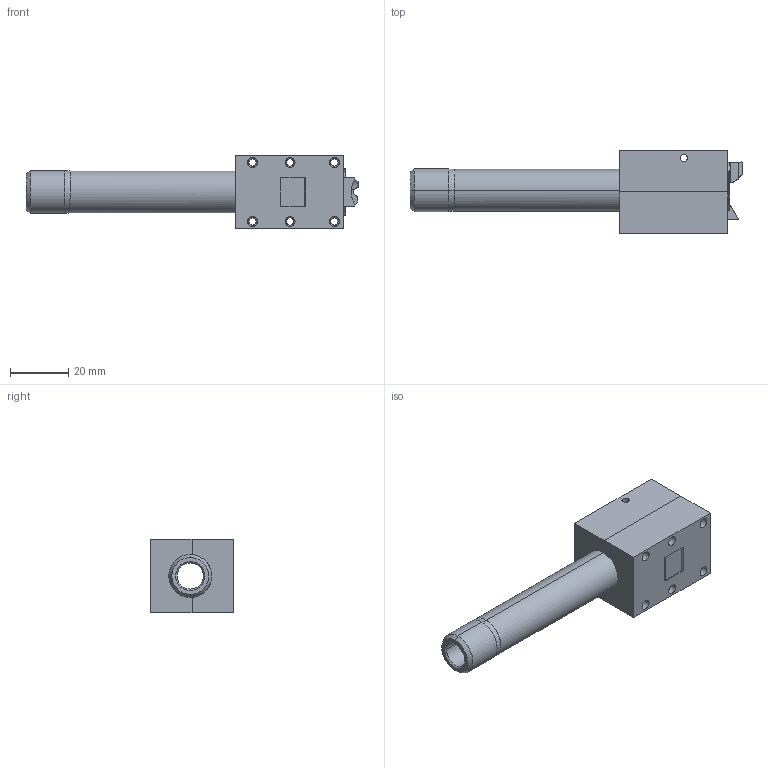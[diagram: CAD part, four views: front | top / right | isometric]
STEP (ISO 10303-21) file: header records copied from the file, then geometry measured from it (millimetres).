
FILE_DESCRIPTION (( 'STEP AP214' ), '1' );
FILE_NAME ('PPDW9 V4 RP9 Barrel and block.STEP', '2020-12-31T18:34:29', ( '' ), ( '' ), 'SwSTEP 2.0', 'SolidWorks 2020', '' );
FILE_SCHEMA (( 'AUTOMOTIVE_DESIGN' ));
Length unit declared in the file: inch
Products named in the file (4): Barrel RP9 Modcat modded; PPDW9 V4 RP9 Barrel and block; Barrel Block V4 RP9 split bottom; Barrel Block V4 RP9 split top
Assembly tree (3 placements, depth 2):
  PPDW9 V4 RP9 Barrel and block
    Barrel RP9 Modcat modded
    Barrel Block V4 RP9 split bottom
    Barrel Block V4 RP9 split top
Bounding box: 114.25 x 28.7 x 25.4 mm (x, y, z)
Volume: 30376.8 mm3; surface area: 19115.1 mm2
Topology: 3 solids, 3 shells, 482 faces, 1293 edges, 828 vertices
Faces by surface type: plane 203, cylinder 131, bspline 100, cone 25, sphere 13, torus 10
Entity records: 19248 total; most frequent: CARTESIAN_POINT 7593, ORIENTED_EDGE 2566, DIRECTION 1998, EDGE_CURVE 1283, VERTEX_POINT 828, LINE 728, VECTOR 728, AXIS2_PLACEMENT_3D 635
